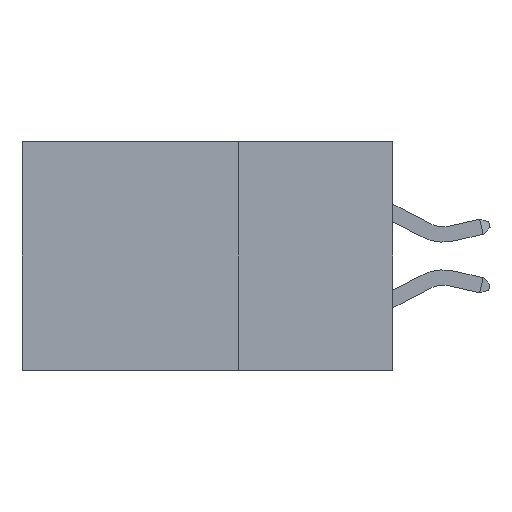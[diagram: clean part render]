
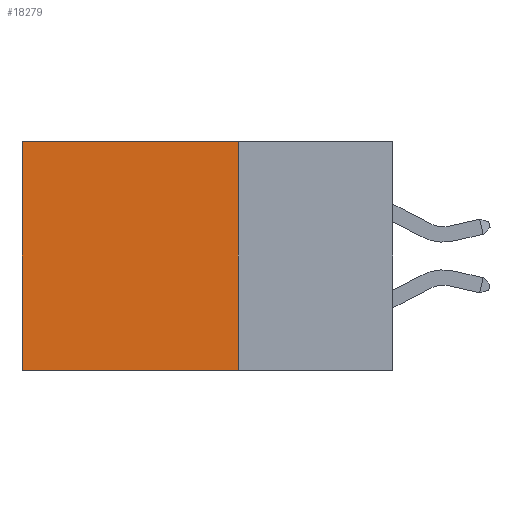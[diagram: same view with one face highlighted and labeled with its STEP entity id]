
A CAD part, left-side view. The second image highlights one B-rep face of the part: STEP entity #18279.
In plain terms, the highlighted planar face has unit normal (-1, 0, 0).
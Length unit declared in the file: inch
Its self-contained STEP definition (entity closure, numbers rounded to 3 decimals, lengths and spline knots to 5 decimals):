
#370 = DIRECTION ( 'NONE',  ( 0., 0., -1. ) ) ;
#511 = CARTESIAN_POINT ( 'NONE',  ( 0.2875, 0.25, 0. ) ) ;
#1691 = EDGE_LOOP ( 'NONE', ( #5077, #21686, #6228, #20622 ) ) ;
#2027 = DIRECTION ( 'NONE',  ( 0., 1., 0. ) ) ;
#2408 = CARTESIAN_POINT ( 'NONE',  ( 0.2875, 0.6, 0. ) ) ;
#3382 = FACE_OUTER_BOUND ( 'NONE', #1691, .T. ) ;
#5077 = ORIENTED_EDGE ( 'NONE', *, *, #7135, .T. ) ;
#5220 = CARTESIAN_POINT ( 'NONE',  ( 0.2875, 0.25, -0.37 ) ) ;
#6228 = ORIENTED_EDGE ( 'NONE', *, *, #23008, .F. ) ;
#6310 = CARTESIAN_POINT ( 'NONE',  ( 0.2875, 0.6, -0.37 ) ) ;
#7022 = EDGE_CURVE ( 'NONE', #14472, #14554, #13243, .T. ) ;
#7135 = EDGE_CURVE ( 'NONE', #18582, #14554, #17817, .T. ) ;
#8957 = VECTOR ( 'NONE', #16044, 39.37008 ) ;
#9109 = DIRECTION ( 'NONE',  ( 0., 0., -1. ) ) ;
#9235 = DIRECTION ( 'NONE',  ( 1., 0., 0. ) ) ;
#10901 = PLANE ( 'NONE',  #24295 ) ;
#12994 = DIRECTION ( 'NONE',  ( 0., 1., 0. ) ) ;
#13243 = LINE ( 'NONE', #5220, #20658 ) ;
#13608 = CARTESIAN_POINT ( 'NONE',  ( 0.2875, 0.25, 0. ) ) ;
#14472 = VERTEX_POINT ( 'NONE', #20194 ) ;
#14554 = VERTEX_POINT ( 'NONE', #6310 ) ;
#16044 = DIRECTION ( 'NONE',  ( 0., 0., -1. ) ) ;
#16102 = VERTEX_POINT ( 'NONE', #19547 ) ;
#17817 = LINE ( 'NONE', #2408, #21890 ) ;
#18279 = ADVANCED_FACE ( 'NONE', ( #3382 ), #10901, .F. ) ;
#18582 = VERTEX_POINT ( 'NONE', #20672 ) ;
#19547 = CARTESIAN_POINT ( 'NONE',  ( 0.2875, 0.25, 0. ) ) ;
#20194 = CARTESIAN_POINT ( 'NONE',  ( 0.2875, 0.25, -0.37 ) ) ;
#20622 = ORIENTED_EDGE ( 'NONE', *, *, #24605, .T. ) ;
#20658 = VECTOR ( 'NONE', #12994, 39.37008 ) ;
#20672 = CARTESIAN_POINT ( 'NONE',  ( 0.2875, 0.6, 0. ) ) ;
#21686 = ORIENTED_EDGE ( 'NONE', *, *, #7022, .F. ) ;
#21890 = VECTOR ( 'NONE', #370, 39.37008 ) ;
#22276 = LINE ( 'NONE', #511, #8957 ) ;
#22746 = CARTESIAN_POINT ( 'NONE',  ( 0.2875, 0.25, 0. ) ) ;
#23008 = EDGE_CURVE ( 'NONE', #16102, #14472, #22276, .T. ) ;
#23296 = LINE ( 'NONE', #13608, #24486 ) ;
#24295 = AXIS2_PLACEMENT_3D ( 'NONE', #22746, #9235, #9109 ) ;
#24486 = VECTOR ( 'NONE', #2027, 39.37008 ) ;
#24605 = EDGE_CURVE ( 'NONE', #16102, #18582, #23296, .T. ) ;
